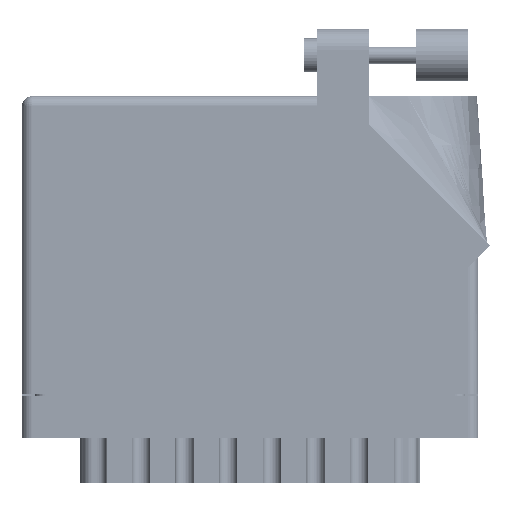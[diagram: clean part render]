
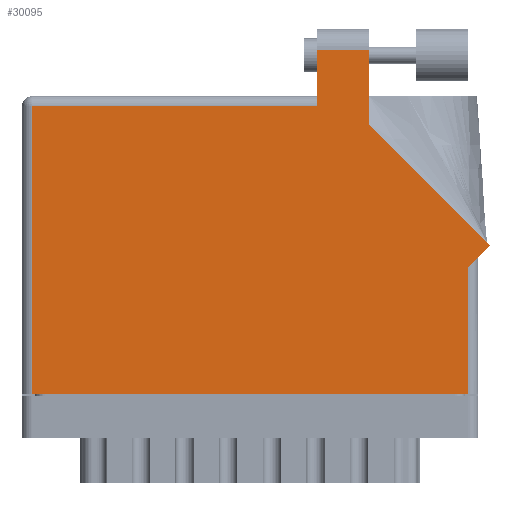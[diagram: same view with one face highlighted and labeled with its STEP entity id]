
A CAD part, front view. The second image highlights one B-rep face of the part: STEP entity #30095.
In plain terms, the highlighted face is planar.
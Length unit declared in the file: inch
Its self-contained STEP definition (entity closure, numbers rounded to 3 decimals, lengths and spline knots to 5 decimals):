
#572 = DIRECTION ( 'NONE',  ( -1., 0., 0. ) ) ;
#3828 = ORIENTED_EDGE ( 'NONE', *, *, #66584, .T. ) ;
#5213 = CARTESIAN_POINT ( 'NONE',  ( 2.065, 2.05, 0. ) ) ;
#5265 = DIRECTION ( 'NONE',  ( 0., 0., -1. ) ) ;
#5341 = VECTOR ( 'NONE', #56920, 39.37008 ) ;
#6560 = DIRECTION ( 'NONE',  ( 0., -1., 0. ) ) ;
#6578 = CARTESIAN_POINT ( 'NONE',  ( 1.758, 2.05, 0. ) ) ;
#6822 = VECTOR ( 'NONE', #70478, 39.37008 ) ;
#9293 = AXIS2_PLACEMENT_3D ( 'NONE', #62506, #5265, #50965 ) ;
#10610 = CARTESIAN_POINT ( 'NONE',  ( 2.78871, 0.88571, 0. ) ) ;
#11711 = LINE ( 'NONE', #6578, #43355 ) ;
#12436 = EDGE_CURVE ( 'NONE', #49038, #64820, #64575, .T. ) ;
#12615 = DIRECTION ( 'NONE',  ( 0., 1., 0. ) ) ;
#12959 = CARTESIAN_POINT ( 'NONE',  ( 2.065, 1.60942, 0. ) ) ;
#14119 = ORIENTED_EDGE ( 'NONE', *, *, #12436, .T. ) ;
#14245 = CARTESIAN_POINT ( 'NONE',  ( 0.062, 0., 0. ) ) ;
#15209 = ORIENTED_EDGE ( 'NONE', *, *, #47577, .T. ) ;
#16635 = VERTEX_POINT ( 'NONE', #32986 ) ;
#17193 = VERTEX_POINT ( 'NONE', #50950 ) ;
#17240 = VECTOR ( 'NONE', #64917, 39.37008 ) ;
#18365 = CARTESIAN_POINT ( 'NONE',  ( 1.758, 1.775, 0. ) ) ;
#20106 = ORIENTED_EDGE ( 'NONE', *, *, #52184, .T. ) ;
#20725 = CARTESIAN_POINT ( 'NONE',  ( 0., 1.713, 0. ) ) ;
#20820 = ORIENTED_EDGE ( 'NONE', *, *, #36483, .T. ) ;
#21771 = LINE ( 'NONE', #65060, #6822 ) ;
#25412 = ORIENTED_EDGE ( 'NONE', *, *, #70415, .T. ) ;
#26232 = CARTESIAN_POINT ( 'NONE',  ( 2.656, 0., 0. ) ) ;
#29003 = VERTEX_POINT ( 'NONE', #56994 ) ;
#30050 = DIRECTION ( 'NONE',  ( 0., -1., 0. ) ) ;
#30095 = ADVANCED_FACE ( 'NONE', ( #31000 ), #45067, .F. ) ;
#30223 = VERTEX_POINT ( 'NONE', #68708 ) ;
#31000 = FACE_OUTER_BOUND ( 'NONE', #51990, .T. ) ;
#32128 = LINE ( 'NONE', #48409, #17240 ) ;
#32475 = VECTOR ( 'NONE', #12615, 39.37008 ) ;
#32986 = CARTESIAN_POINT ( 'NONE',  ( 2.656, 0.753, 0. ) ) ;
#36033 = VERTEX_POINT ( 'NONE', #14245 ) ;
#36160 = LINE ( 'NONE', #18365, #67880 ) ;
#36483 = EDGE_CURVE ( 'NONE', #65765, #30223, #11711, .T. ) ;
#38110 = LINE ( 'NONE', #63786, #60131 ) ;
#41098 = CARTESIAN_POINT ( 'NONE',  ( 2.78871, 0.88571, 0. ) ) ;
#42389 = EDGE_CURVE ( 'NONE', #29003, #36033, #38110, .T. ) ;
#43355 = VECTOR ( 'NONE', #572, 39.37008 ) ;
#45067 = PLANE ( 'NONE',  #9293 ) ;
#46496 = DIRECTION ( 'NONE',  ( -0.707, 0.707, 0. ) ) ;
#46709 = CARTESIAN_POINT ( 'NONE',  ( 2.065, 1.60942, 0. ) ) ;
#47577 = EDGE_CURVE ( 'NONE', #36033, #47773, #32128, .T. ) ;
#47773 = VERTEX_POINT ( 'NONE', #26232 ) ;
#48409 = CARTESIAN_POINT ( 'NONE',  ( 0., 0., 0. ) ) ;
#49038 = VERTEX_POINT ( 'NONE', #10610 ) ;
#49127 = ORIENTED_EDGE ( 'NONE', *, *, #42389, .T. ) ;
#49586 = VECTOR ( 'NONE', #46496, 39.37008 ) ;
#50950 = CARTESIAN_POINT ( 'NONE',  ( 1.758, 1.713, 0. ) ) ;
#50965 = DIRECTION ( 'NONE',  ( -1., 0., 0. ) ) ;
#51990 = EDGE_LOOP ( 'NONE', ( #64919, #20820, #20106, #66862, #49127, #15209, #3828, #25412, #14119 ) ) ;
#52184 = EDGE_CURVE ( 'NONE', #30223, #17193, #36160, .T. ) ;
#53440 = EDGE_CURVE ( 'NONE', #64820, #65765, #62405, .T. ) ;
#54367 = DIRECTION ( 'NONE',  ( -1., 0., 0. ) ) ;
#55472 = LINE ( 'NONE', #68560, #5341 ) ;
#56920 = DIRECTION ( 'NONE',  ( 0., 1., 0. ) ) ;
#56994 = CARTESIAN_POINT ( 'NONE',  ( 0.062, 1.713, 0. ) ) ;
#60131 = VECTOR ( 'NONE', #30050, 39.37008 ) ;
#61431 = LINE ( 'NONE', #20725, #65016 ) ;
#62405 = LINE ( 'NONE', #46709, #32475 ) ;
#62506 = CARTESIAN_POINT ( 'NONE',  ( 0., 1.775, 0. ) ) ;
#63786 = CARTESIAN_POINT ( 'NONE',  ( 0.062, 0., 0. ) ) ;
#64575 = LINE ( 'NONE', #41098, #49586 ) ;
#64820 = VERTEX_POINT ( 'NONE', #12959 ) ;
#64917 = DIRECTION ( 'NONE',  ( 1., 0., 0. ) ) ;
#64919 = ORIENTED_EDGE ( 'NONE', *, *, #53440, .T. ) ;
#65016 = VECTOR ( 'NONE', #54367, 39.37008 ) ;
#65060 = CARTESIAN_POINT ( 'NONE',  ( 2.718, 0.815, 0. ) ) ;
#65765 = VERTEX_POINT ( 'NONE', #5213 ) ;
#66584 = EDGE_CURVE ( 'NONE', #47773, #16635, #55472, .T. ) ;
#66862 = ORIENTED_EDGE ( 'NONE', *, *, #69184, .T. ) ;
#67880 = VECTOR ( 'NONE', #6560, 39.37008 ) ;
#68560 = CARTESIAN_POINT ( 'NONE',  ( 2.656, 0.815, 0. ) ) ;
#68708 = CARTESIAN_POINT ( 'NONE',  ( 1.758, 2.05, 0. ) ) ;
#69184 = EDGE_CURVE ( 'NONE', #17193, #29003, #61431, .T. ) ;
#70415 = EDGE_CURVE ( 'NONE', #16635, #49038, #21771, .T. ) ;
#70478 = DIRECTION ( 'NONE',  ( 0.707, 0.707, 0. ) ) ;
